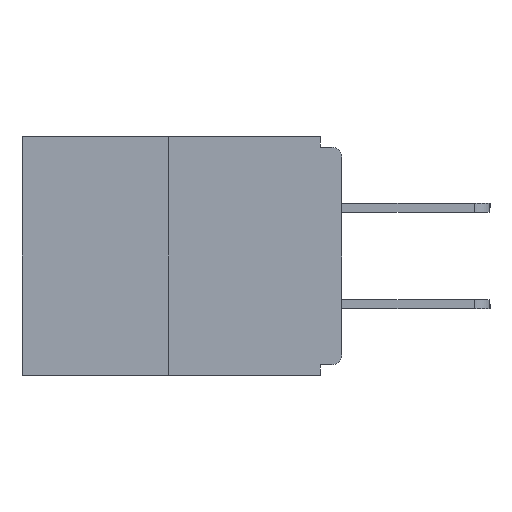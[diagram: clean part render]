
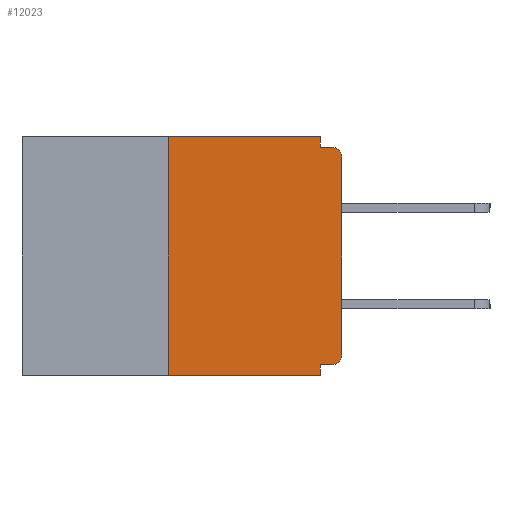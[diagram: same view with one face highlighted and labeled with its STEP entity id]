
A CAD part, left-side view. The second image highlights one B-rep face of the part: STEP entity #12023.
In plain terms, the highlighted planar face has unit normal (-1, 0, 0).
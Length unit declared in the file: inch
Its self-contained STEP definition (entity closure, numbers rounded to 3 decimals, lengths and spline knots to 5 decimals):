
#80 = AXIS2_PLACEMENT_3D ( 'NONE', #10894, #3787, #6905 ) ;
#353 = CARTESIAN_POINT ( 'NONE',  ( 0., 0., -0.328 ) ) ;
#414 = ORIENTED_EDGE ( 'NONE', *, *, #8034, .F. ) ;
#757 = VECTOR ( 'NONE', #9316, 39.37008 ) ;
#770 = VECTOR ( 'NONE', #3897, 39.37008 ) ;
#912 = EDGE_CURVE ( 'NONE', #10597, #3331, #9783, .T. ) ;
#1053 = LINE ( 'NONE', #11768, #11955 ) ;
#1071 = LINE ( 'NONE', #11051, #770 ) ;
#1240 = DIRECTION ( 'NONE',  ( 0., 0., -1. ) ) ;
#1250 = CARTESIAN_POINT ( 'NONE',  ( 0., 0., -0.313 ) ) ;
#1285 = CARTESIAN_POINT ( 'NONE',  ( 0., 0.46, 0. ) ) ;
#1591 = CARTESIAN_POINT ( 'NONE',  ( 0., 0.25, -0.343 ) ) ;
#2595 = EDGE_CURVE ( 'NONE', #5631, #3491, #3894, .T. ) ;
#2801 = AXIS2_PLACEMENT_3D ( 'NONE', #1285, #7311, #1240 ) ;
#3090 = ORIENTED_EDGE ( 'NONE', *, *, #9085, .T. ) ;
#3220 = EDGE_CURVE ( 'NONE', #3331, #5512, #5809, .T. ) ;
#3232 = LINE ( 'NONE', #353, #11313 ) ;
#3248 = VECTOR ( 'NONE', #10729, 39.37008 ) ;
#3331 = VERTEX_POINT ( 'NONE', #12840 ) ;
#3356 = VERTEX_POINT ( 'NONE', #5636 ) ;
#3491 = VERTEX_POINT ( 'NONE', #9018 ) ;
#3662 = CARTESIAN_POINT ( 'NONE',  ( 0., 0., 0. ) ) ;
#3787 = DIRECTION ( 'NONE',  ( -1., 0., 0. ) ) ;
#3817 = ORIENTED_EDGE ( 'NONE', *, *, #10538, .F. ) ;
#3894 = LINE ( 'NONE', #3662, #3248 ) ;
#3897 = DIRECTION ( 'NONE',  ( 0., -1., 0. ) ) ;
#3958 = CARTESIAN_POINT ( 'NONE',  ( 0., 0.25, 0. ) ) ;
#4064 = LINE ( 'NONE', #11308, #757 ) ;
#4246 = CARTESIAN_POINT ( 'NONE',  ( 0., 0.031, 0. ) ) ;
#4643 = CARTESIAN_POINT ( 'NONE',  ( 0., 0.015, -0.313 ) ) ;
#4658 = EDGE_CURVE ( 'NONE', #8120, #5631, #10315, .T. ) ;
#4709 = CARTESIAN_POINT ( 'NONE',  ( 0., 0.25, 0. ) ) ;
#4849 = CARTESIAN_POINT ( 'NONE',  ( 0., 0.015, -0.015 ) ) ;
#5512 = VERTEX_POINT ( 'NONE', #4849 ) ;
#5631 = VERTEX_POINT ( 'NONE', #1250 ) ;
#5636 = CARTESIAN_POINT ( 'NONE',  ( 0., 0.031, -0.328 ) ) ;
#5794 = DIRECTION ( 'NONE',  ( 0., 0., 1. ) ) ;
#5809 = LINE ( 'NONE', #7504, #8018 ) ;
#6056 = ORIENTED_EDGE ( 'NONE', *, *, #9949, .F. ) ;
#6366 = EDGE_CURVE ( 'NONE', #7075, #11329, #6501, .T. ) ;
#6501 = LINE ( 'NONE', #4709, #10272 ) ;
#6566 = DIRECTION ( 'NONE',  ( 0., 0., -1. ) ) ;
#6597 = DIRECTION ( 'NONE',  ( 0., -1., 0. ) ) ;
#6601 = CARTESIAN_POINT ( 'NONE',  ( 0., 0.031, 0. ) ) ;
#6905 = DIRECTION ( 'NONE',  ( 0., 0., -1. ) ) ;
#6926 = CARTESIAN_POINT ( 'NONE',  ( 0., 0.031, -0.343 ) ) ;
#7075 = VERTEX_POINT ( 'NONE', #1591 ) ;
#7183 = PLANE ( 'NONE',  #2801 ) ;
#7311 = DIRECTION ( 'NONE',  ( 1., 0., 0. ) ) ;
#7347 = ORIENTED_EDGE ( 'NONE', *, *, #6366, .F. ) ;
#7504 = CARTESIAN_POINT ( 'NONE',  ( 0., 0., -0.015 ) ) ;
#7536 = DIRECTION ( 'NONE',  ( 0., 1., 0. ) ) ;
#7918 = ORIENTED_EDGE ( 'NONE', *, *, #912, .F. ) ;
#8018 = VECTOR ( 'NONE', #6597, 39.37008 ) ;
#8034 = EDGE_CURVE ( 'NONE', #11329, #10597, #1071, .T. ) ;
#8120 = VERTEX_POINT ( 'NONE', #11186 ) ;
#8459 = FACE_OUTER_BOUND ( 'NONE', #9731, .T. ) ;
#9018 = CARTESIAN_POINT ( 'NONE',  ( 0., 0., -0.03 ) ) ;
#9085 = EDGE_CURVE ( 'NONE', #7075, #11835, #4064, .T. ) ;
#9316 = DIRECTION ( 'NONE',  ( 0., -1., 0. ) ) ;
#9430 = AXIS2_PLACEMENT_3D ( 'NONE', #4643, #9727, #11793 ) ;
#9727 = DIRECTION ( 'NONE',  ( -1., 0., 0. ) ) ;
#9731 = EDGE_LOOP ( 'NONE', ( #414, #7347, #3090, #6056, #3817, #12606, #12095, #11766, #9994, #7918 ) ) ;
#9783 = LINE ( 'NONE', #6601, #13105 ) ;
#9949 = EDGE_CURVE ( 'NONE', #3356, #11835, #1053, .T. ) ;
#9994 = ORIENTED_EDGE ( 'NONE', *, *, #3220, .F. ) ;
#10272 = VECTOR ( 'NONE', #5794, 39.37008 ) ;
#10311 = EDGE_CURVE ( 'NONE', #3491, #5512, #13058, .T. ) ;
#10315 = CIRCLE ( 'NONE', #9430, 0.015 ) ;
#10538 = EDGE_CURVE ( 'NONE', #8120, #3356, #3232, .T. ) ;
#10597 = VERTEX_POINT ( 'NONE', #4246 ) ;
#10729 = DIRECTION ( 'NONE',  ( 0., 0., 1. ) ) ;
#10894 = CARTESIAN_POINT ( 'NONE',  ( 0., 0.015, -0.03 ) ) ;
#11051 = CARTESIAN_POINT ( 'NONE',  ( 0., 0.46, 0. ) ) ;
#11186 = CARTESIAN_POINT ( 'NONE',  ( 0., 0.015, -0.328 ) ) ;
#11308 = CARTESIAN_POINT ( 'NONE',  ( 0., 0.46, -0.343 ) ) ;
#11313 = VECTOR ( 'NONE', #7536, 39.37008 ) ;
#11329 = VERTEX_POINT ( 'NONE', #3958 ) ;
#11766 = ORIENTED_EDGE ( 'NONE', *, *, #10311, .T. ) ;
#11768 = CARTESIAN_POINT ( 'NONE',  ( 0., 0.031, -0.343 ) ) ;
#11793 = DIRECTION ( 'NONE',  ( 0., 0., -1. ) ) ;
#11835 = VERTEX_POINT ( 'NONE', #6926 ) ;
#11955 = VECTOR ( 'NONE', #6566, 39.37008 ) ;
#12023 = ADVANCED_FACE ( 'NONE', ( #8459 ), #7183, .F. ) ;
#12095 = ORIENTED_EDGE ( 'NONE', *, *, #2595, .T. ) ;
#12606 = ORIENTED_EDGE ( 'NONE', *, *, #4658, .T. ) ;
#12610 = DIRECTION ( 'NONE',  ( 0., 0., -1. ) ) ;
#12840 = CARTESIAN_POINT ( 'NONE',  ( 0., 0.031, -0.015 ) ) ;
#13058 = CIRCLE ( 'NONE', #80, 0.015 ) ;
#13105 = VECTOR ( 'NONE', #12610, 39.37008 ) ;
